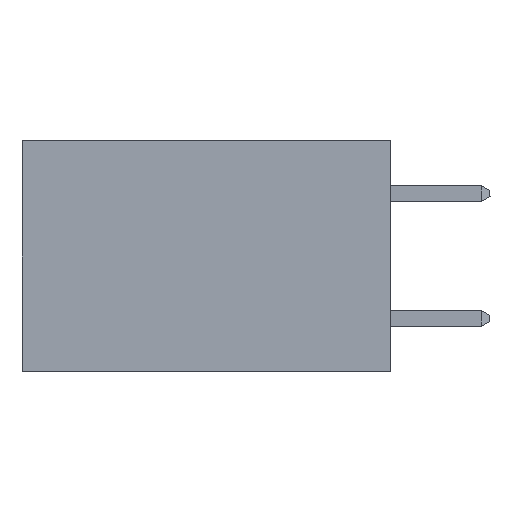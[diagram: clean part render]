
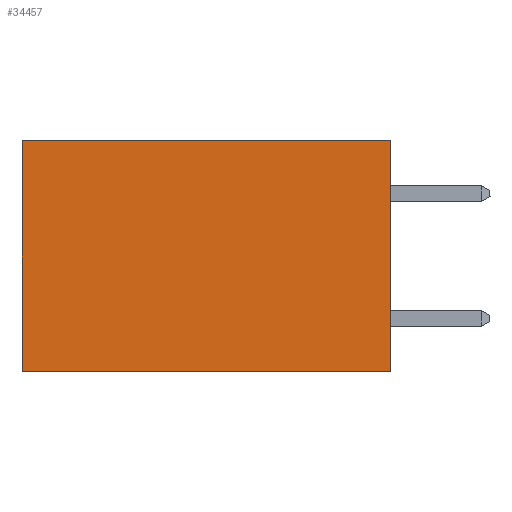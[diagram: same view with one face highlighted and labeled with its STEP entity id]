
A CAD part, left-side view. The second image highlights one B-rep face of the part: STEP entity #34457.
In plain terms, the highlighted planar face has unit normal (-1, 0, 0).
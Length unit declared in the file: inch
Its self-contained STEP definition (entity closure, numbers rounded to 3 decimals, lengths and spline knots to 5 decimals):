
#535 = DIRECTION ( 'NONE',  ( 1., 0., 0. ) ) ;
#3190 = VERTEX_POINT ( 'NONE', #17609 ) ;
#4215 = CARTESIAN_POINT ( 'NONE',  ( 0.277, 0.59, -0.37 ) ) ;
#5769 = VERTEX_POINT ( 'NONE', #4215 ) ;
#6351 = ORIENTED_EDGE ( 'NONE', *, *, #23288, .F. ) ;
#6677 = AXIS2_PLACEMENT_3D ( 'NONE', #19416, #535, #19537 ) ;
#6917 = VECTOR ( 'NONE', #18225, 39.37008 ) ;
#7599 = VECTOR ( 'NONE', #29332, 39.37008 ) ;
#8136 = ORIENTED_EDGE ( 'NONE', *, *, #25834, .T. ) ;
#8570 = CARTESIAN_POINT ( 'NONE',  ( 0.277, 0., -0.37 ) ) ;
#9882 = CARTESIAN_POINT ( 'NONE',  ( 0.277, 0., -0.37 ) ) ;
#12573 = DIRECTION ( 'NONE',  ( 0., 0., -1. ) ) ;
#12616 = DIRECTION ( 'NONE',  ( 0., 1., 0. ) ) ;
#14414 = EDGE_LOOP ( 'NONE', ( #8136, #18452, #6351, #15116 ) ) ;
#14786 = LINE ( 'NONE', #29215, #7599 ) ;
#15116 = ORIENTED_EDGE ( 'NONE', *, *, #34226, .T. ) ;
#15207 = FACE_OUTER_BOUND ( 'NONE', #14414, .T. ) ;
#15505 = CARTESIAN_POINT ( 'NONE',  ( 0.277, 0.59, -0.37 ) ) ;
#16144 = VERTEX_POINT ( 'NONE', #32619 ) ;
#17609 = CARTESIAN_POINT ( 'NONE',  ( 0.277, 0., 0. ) ) ;
#18225 = DIRECTION ( 'NONE',  ( 0., 0., -1. ) ) ;
#18452 = ORIENTED_EDGE ( 'NONE', *, *, #24393, .F. ) ;
#19230 = LINE ( 'NONE', #9882, #25503 ) ;
#19416 = CARTESIAN_POINT ( 'NONE',  ( 0.277, 0., -0.37 ) ) ;
#19537 = DIRECTION ( 'NONE',  ( 0., 0., -1. ) ) ;
#23288 = EDGE_CURVE ( 'NONE', #3190, #33668, #19230, .T. ) ;
#24393 = EDGE_CURVE ( 'NONE', #33668, #5769, #34313, .T. ) ;
#25503 = VECTOR ( 'NONE', #12573, 39.37008 ) ;
#25834 = EDGE_CURVE ( 'NONE', #16144, #5769, #28344, .T. ) ;
#26019 = CARTESIAN_POINT ( 'NONE',  ( 0.277, 0., -0.37 ) ) ;
#28344 = LINE ( 'NONE', #15505, #6917 ) ;
#29215 = CARTESIAN_POINT ( 'NONE',  ( 0.277, 0., 0. ) ) ;
#29332 = DIRECTION ( 'NONE',  ( 0., 1., 0. ) ) ;
#32619 = CARTESIAN_POINT ( 'NONE',  ( 0.277, 0.59, 0. ) ) ;
#32653 = VECTOR ( 'NONE', #12616, 39.37008 ) ;
#32838 = PLANE ( 'NONE',  #6677 ) ;
#33668 = VERTEX_POINT ( 'NONE', #8570 ) ;
#34226 = EDGE_CURVE ( 'NONE', #3190, #16144, #14786, .T. ) ;
#34313 = LINE ( 'NONE', #26019, #32653 ) ;
#34457 = ADVANCED_FACE ( 'NONE', ( #15207 ), #32838, .F. ) ;
